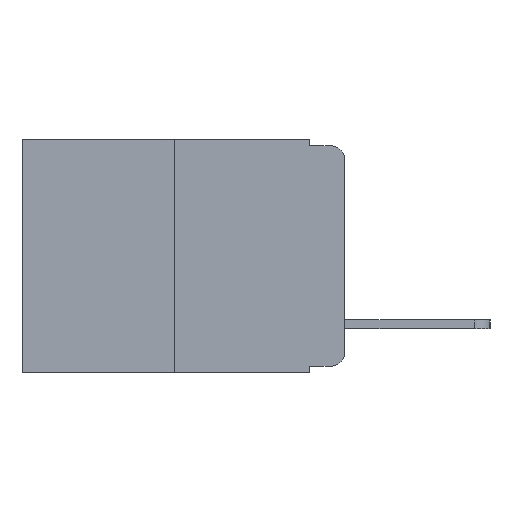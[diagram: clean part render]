
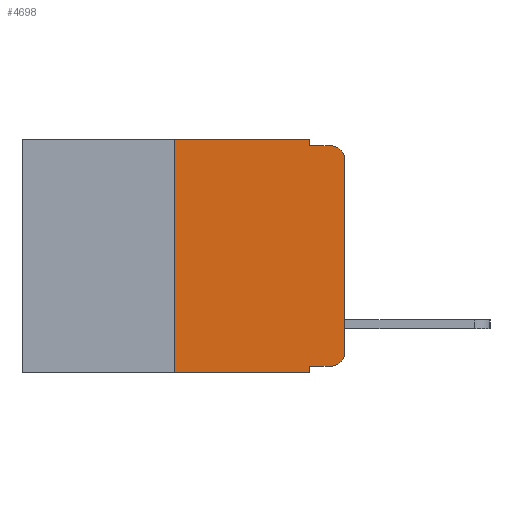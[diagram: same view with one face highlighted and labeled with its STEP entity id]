
A CAD part, left-side view. The second image highlights one B-rep face of the part: STEP entity #4698.
In plain terms, the highlighted planar face has unit normal (-1, 0, 0).
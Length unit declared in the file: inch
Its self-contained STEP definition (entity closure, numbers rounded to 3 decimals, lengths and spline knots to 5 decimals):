
#53 = ORIENTED_EDGE ( 'NONE', *, *, #12338, .T. ) ;
#268 = ORIENTED_EDGE ( 'NONE', *, *, #3077, .F. ) ;
#530 = CARTESIAN_POINT ( 'NONE',  ( 0., 0.051, -0.333 ) ) ;
#683 = VECTOR ( 'NONE', #15931, 39.37008 ) ;
#825 = EDGE_CURVE ( 'NONE', #7551, #9798, #19156, .T. ) ;
#982 = VERTEX_POINT ( 'NONE', #17719 ) ;
#1645 = EDGE_CURVE ( 'NONE', #982, #16004, #8950, .T. ) ;
#1769 = EDGE_CURVE ( 'NONE', #8498, #3616, #3017, .T. ) ;
#1894 = CARTESIAN_POINT ( 'NONE',  ( 0., 0.02, -0.03 ) ) ;
#1942 = CARTESIAN_POINT ( 'NONE',  ( 0., 0.473, 0. ) ) ;
#2764 = DIRECTION ( 'NONE',  ( 0., 0., -1. ) ) ;
#2956 = LINE ( 'NONE', #3376, #14432 ) ;
#3017 = CIRCLE ( 'NONE', #11232, 0.02 ) ;
#3077 = EDGE_CURVE ( 'NONE', #9795, #982, #2956, .T. ) ;
#3162 = VERTEX_POINT ( 'NONE', #530 ) ;
#3376 = CARTESIAN_POINT ( 'NONE',  ( 0., 0.473, 0. ) ) ;
#3400 = ORIENTED_EDGE ( 'NONE', *, *, #4865, .F. ) ;
#3511 = PLANE ( 'NONE',  #19018 ) ;
#3616 = VERTEX_POINT ( 'NONE', #4746 ) ;
#3859 = CARTESIAN_POINT ( 'NONE',  ( 0., 0.25, -0.343 ) ) ;
#4051 = LINE ( 'NONE', #8736, #11535 ) ;
#4439 = VECTOR ( 'NONE', #19252, 39.37008 ) ;
#4698 = ADVANCED_FACE ( 'NONE', ( #8075 ), #3511, .F. ) ;
#4746 = CARTESIAN_POINT ( 'NONE',  ( 0., 0.02, -0.01 ) ) ;
#4865 = EDGE_CURVE ( 'NONE', #16004, #3616, #14115, .T. ) ;
#4885 = VERTEX_POINT ( 'NONE', #8597 ) ;
#6068 = CARTESIAN_POINT ( 'NONE',  ( 0., 0., -0.03 ) ) ;
#6256 = ORIENTED_EDGE ( 'NONE', *, *, #13720, .F. ) ;
#6421 = EDGE_CURVE ( 'NONE', #7551, #9795, #14753, .T. ) ;
#6436 = DIRECTION ( 'NONE',  ( 0., -1., 0. ) ) ;
#6881 = DIRECTION ( 'NONE',  ( 0., -1., 0. ) ) ;
#7117 = CARTESIAN_POINT ( 'NONE',  ( 0., 0., 0. ) ) ;
#7179 = ORIENTED_EDGE ( 'NONE', *, *, #18628, .T. ) ;
#7263 = CARTESIAN_POINT ( 'NONE',  ( 0., 0.02, -0.313 ) ) ;
#7551 = VERTEX_POINT ( 'NONE', #3859 ) ;
#7962 = CARTESIAN_POINT ( 'NONE',  ( 0., 0.051, 0. ) ) ;
#8065 = DIRECTION ( 'NONE',  ( 1., 0., 0. ) ) ;
#8075 = FACE_OUTER_BOUND ( 'NONE', #18289, .T. ) ;
#8183 = CARTESIAN_POINT ( 'NONE',  ( 0., 0.051, -0.01 ) ) ;
#8190 = CIRCLE ( 'NONE', #17312, 0.02 ) ;
#8498 = VERTEX_POINT ( 'NONE', #6068 ) ;
#8597 = CARTESIAN_POINT ( 'NONE',  ( 0., 0., -0.313 ) ) ;
#8736 = CARTESIAN_POINT ( 'NONE',  ( 0., 0.051, 0. ) ) ;
#8798 = DIRECTION ( 'NONE',  ( 0., 0., -1. ) ) ;
#8950 = LINE ( 'NONE', #7962, #4439 ) ;
#9700 = CARTESIAN_POINT ( 'NONE',  ( 0., 0.25, 0. ) ) ;
#9795 = VERTEX_POINT ( 'NONE', #15947 ) ;
#9798 = VERTEX_POINT ( 'NONE', #13085 ) ;
#10110 = DIRECTION ( 'NONE',  ( 0., 0., -1. ) ) ;
#10676 = VECTOR ( 'NONE', #6881, 39.37008 ) ;
#10729 = DIRECTION ( 'NONE',  ( -1., 0., 0. ) ) ;
#11151 = VERTEX_POINT ( 'NONE', #16695 ) ;
#11168 = DIRECTION ( 'NONE',  ( 0., 0., 1. ) ) ;
#11232 = AXIS2_PLACEMENT_3D ( 'NONE', #1894, #10729, #10110 ) ;
#11535 = VECTOR ( 'NONE', #2764, 39.37008 ) ;
#11817 = ORIENTED_EDGE ( 'NONE', *, *, #1645, .F. ) ;
#12338 = EDGE_CURVE ( 'NONE', #11151, #4885, #8190, .T. ) ;
#12786 = ORIENTED_EDGE ( 'NONE', *, *, #6421, .F. ) ;
#13085 = CARTESIAN_POINT ( 'NONE',  ( 0., 0.051, -0.343 ) ) ;
#13720 = EDGE_CURVE ( 'NONE', #3162, #9798, #4051, .T. ) ;
#13761 = VECTOR ( 'NONE', #16047, 39.37008 ) ;
#13933 = ORIENTED_EDGE ( 'NONE', *, *, #16183, .T. ) ;
#14115 = LINE ( 'NONE', #18809, #683 ) ;
#14392 = ORIENTED_EDGE ( 'NONE', *, *, #1769, .T. ) ;
#14432 = VECTOR ( 'NONE', #6436, 39.37008 ) ;
#14608 = LINE ( 'NONE', #15806, #10676 ) ;
#14753 = LINE ( 'NONE', #9700, #19090 ) ;
#15806 = CARTESIAN_POINT ( 'NONE',  ( 0., 0.051, -0.333 ) ) ;
#15931 = DIRECTION ( 'NONE',  ( 0., -1., 0. ) ) ;
#15947 = CARTESIAN_POINT ( 'NONE',  ( 0., 0.25, 0. ) ) ;
#16004 = VERTEX_POINT ( 'NONE', #8183 ) ;
#16047 = DIRECTION ( 'NONE',  ( 0., 0., 1. ) ) ;
#16183 = EDGE_CURVE ( 'NONE', #4885, #8498, #17645, .T. ) ;
#16695 = CARTESIAN_POINT ( 'NONE',  ( 0., 0.02, -0.333 ) ) ;
#16699 = CARTESIAN_POINT ( 'NONE',  ( 0., 0.473, -0.343 ) ) ;
#17054 = DIRECTION ( 'NONE',  ( 0., -1., 0. ) ) ;
#17135 = ORIENTED_EDGE ( 'NONE', *, *, #825, .T. ) ;
#17312 = AXIS2_PLACEMENT_3D ( 'NONE', #7263, #17596, #8798 ) ;
#17596 = DIRECTION ( 'NONE',  ( -1., 0., 0. ) ) ;
#17645 = LINE ( 'NONE', #7117, #13761 ) ;
#17719 = CARTESIAN_POINT ( 'NONE',  ( 0., 0.051, 0. ) ) ;
#18289 = EDGE_LOOP ( 'NONE', ( #13933, #14392, #3400, #11817, #268, #12786, #17135, #6256, #7179, #53 ) ) ;
#18381 = DIRECTION ( 'NONE',  ( 0., 0., -1. ) ) ;
#18628 = EDGE_CURVE ( 'NONE', #3162, #11151, #14608, .T. ) ;
#18708 = VECTOR ( 'NONE', #17054, 39.37008 ) ;
#18809 = CARTESIAN_POINT ( 'NONE',  ( 0., 0.051, -0.01 ) ) ;
#19018 = AXIS2_PLACEMENT_3D ( 'NONE', #1942, #8065, #18381 ) ;
#19090 = VECTOR ( 'NONE', #11168, 39.37008 ) ;
#19156 = LINE ( 'NONE', #16699, #18708 ) ;
#19252 = DIRECTION ( 'NONE',  ( 0., 0., -1. ) ) ;
